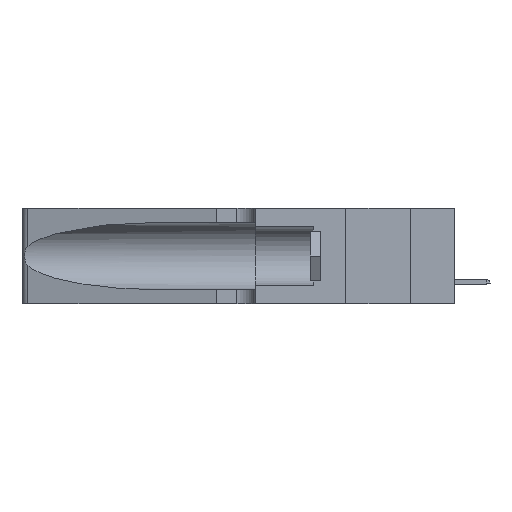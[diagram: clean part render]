
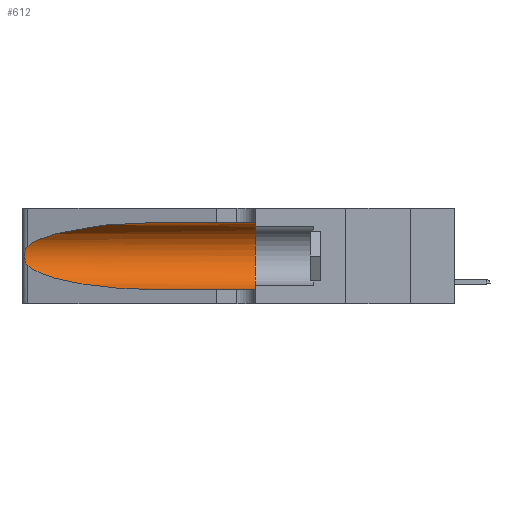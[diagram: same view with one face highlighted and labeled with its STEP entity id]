
A CAD part, left-side view. The second image highlights one B-rep face of the part: STEP entity #612.
In plain terms, the highlighted cylindrical face has radius 3.308 mm (diameter 6.617 mm), a partial arc.
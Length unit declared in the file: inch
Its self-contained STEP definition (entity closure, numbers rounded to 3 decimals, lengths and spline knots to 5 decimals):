
#334 = CARTESIAN_POINT ( 'NONE',  ( 0.26018, 1.23835, 0.19895 ) ) ;
#444 = CYLINDRICAL_SURFACE ( 'NONE', #19863, 0.13025 ) ;
#612 = ADVANCED_FACE ( 'NONE', ( #15831 ), #444, .F. ) ;
#922 = CARTESIAN_POINT ( 'NONE',  ( 0.25555, 1.22993, 0.14849 ) ) ;
#1124 = CARTESIAN_POINT ( 'NONE',  ( 0.25639, 1.23186, 0.15144 ) ) ;
#1495 = CARTESIAN_POINT ( 'NONE',  ( 0.18966, 0.96281, 0.05475 ) ) ;
#1857 = CARTESIAN_POINT ( 'NONE',  ( 0.25854, 1.2359, 0.20912 ) ) ;
#2413 = DIRECTION ( 'NONE',  ( 0., -1., 0. ) ) ;
#3185 = EDGE_CURVE ( 'NONE', #13664, #7599, #10979, .T. ) ;
#4632 = DIRECTION ( 'NONE',  ( 0., 0., -1. ) ) ;
#4920 = EDGE_CURVE ( 'NONE', #14132, #12364, #19684, .T. ) ;
#5044 = CARTESIAN_POINT ( 'NONE',  ( 0.26075, 1.23896, 0.178 ) ) ;
#5285 = CARTESIAN_POINT ( 'NONE',  ( 0.18966, 0.96281, 0.31525 ) ) ;
#5530 = ORIENTED_EDGE ( 'NONE', *, *, #4920, .T. ) ;
#5553 = VECTOR ( 'NONE', #2413, 39.37008 ) ;
#5659 =( BOUNDED_CURVE ( )  B_SPLINE_CURVE ( 3, ( #7695, #5937, #1495, #12233 ),
 .UNSPECIFIED., .F., .F. ) 
 B_SPLINE_CURVE_WITH_KNOTS ( ( 4, 4 ),
 ( 3.44316, 4.71239 ),
 .UNSPECIFIED. ) 
 CURVE ( )  GEOMETRIC_REPRESENTATION_ITEM ( )  RATIONAL_B_SPLINE_CURVE ( ( 1., 0.87, 0.87, 1. ) ) 
 REPRESENTATION_ITEM ( '' )  );
#5937 = CARTESIAN_POINT ( 'NONE',  ( 0.2373, 1.15595, 0.08982 ) ) ;
#6604 = CARTESIAN_POINT ( 'NONE',  ( 0.26075, 1.23896, 0.19203 ) ) ;
#6623 = ORIENTED_EDGE ( 'NONE', *, *, #3185, .F. ) ;
#6939 = CARTESIAN_POINT ( 'NONE',  ( 0.2373, 1.15595, 0.28018 ) ) ;
#7080 = VERTEX_POINT ( 'NONE', #13266 ) ;
#7240 = ORIENTED_EDGE ( 'NONE', *, *, #14362, .T. ) ;
#7599 = VERTEX_POINT ( 'NONE', #12850 ) ;
#7695 = CARTESIAN_POINT ( 'NONE',  ( 0.25487, 1.22718, 0.14631 ) ) ;
#7906 = ORIENTED_EDGE ( 'NONE', *, *, #10298, .T. ) ;
#8017 = AXIS2_PLACEMENT_3D ( 'NONE', #13587, #19824, #10641 ) ;
#8068 = CARTESIAN_POINT ( 'NONE',  ( 0.1305, 1.61858, 0.185 ) ) ;
#9756 = VERTEX_POINT ( 'NONE', #18602 ) ;
#9932 = CARTESIAN_POINT ( 'NONE',  ( 0.25555, 1.22994, 0.2215 ) ) ;
#10061 = CARTESIAN_POINT ( 'NONE',  ( 0.25487, 1.22718, 0.22369 ) ) ;
#10298 = EDGE_CURVE ( 'NONE', #12364, #9756, #18409, .T. ) ;
#10338 = ORIENTED_EDGE ( 'NONE', *, *, #15326, .T. ) ;
#10390 = CARTESIAN_POINT ( 'NONE',  ( 0.1305, 1.61858, 0.05475 ) ) ;
#10522 = LINE ( 'NONE', #19706, #20082 ) ;
#10641 = DIRECTION ( 'NONE',  ( 0., 0., 1. ) ) ;
#10655 = CARTESIAN_POINT ( 'NONE',  ( 0.25487, 1.22718, 0.14631 ) ) ;
#10979 = CIRCLE ( 'NONE', #8017, 0.13025 ) ;
#11494 = CARTESIAN_POINT ( 'NONE',  ( 0.1305, 0.72297, 0.31525 ) ) ;
#11836 = DIRECTION ( 'NONE',  ( 0., -1., 0. ) ) ;
#11866 = CARTESIAN_POINT ( 'NONE',  ( 0.25856, 1.23593, 0.16098 ) ) ;
#12233 = CARTESIAN_POINT ( 'NONE',  ( 0.1305, 0.72297, 0.05475 ) ) ;
#12364 = VERTEX_POINT ( 'NONE', #16515 ) ;
#12544 = CARTESIAN_POINT ( 'NONE',  ( 0.1305, 0.35, 0.31525 ) ) ;
#12850 = CARTESIAN_POINT ( 'NONE',  ( 0.1305, 0.35, 0.05475 ) ) ;
#13184 = CARTESIAN_POINT ( 'NONE',  ( 0.25787, 1.23484, 0.2124 ) ) ;
#13266 = CARTESIAN_POINT ( 'NONE',  ( 0.1305, 0.72297, 0.05475 ) ) ;
#13587 = CARTESIAN_POINT ( 'NONE',  ( 0.1305, 0.35, 0.185 ) ) ;
#13664 = VERTEX_POINT ( 'NONE', #12544 ) ;
#13961 = EDGE_CURVE ( 'NONE', #14132, #13664, #10522, .T. ) ;
#14132 = VERTEX_POINT ( 'NONE', #17641 ) ;
#14362 = EDGE_CURVE ( 'NONE', #7080, #7599, #19481, .T. ) ;
#15066 = CARTESIAN_POINT ( 'NONE',  ( 0.25789, 1.23486, 0.15765 ) ) ;
#15326 = EDGE_CURVE ( 'NONE', #9756, #7080, #5659, .T. ) ;
#15831 = FACE_OUTER_BOUND ( 'NONE', #17418, .T. ) ;
#16039 = CARTESIAN_POINT ( 'NONE',  ( 0.25487, 1.22718, 0.22369 ) ) ;
#16515 = CARTESIAN_POINT ( 'NONE',  ( 0.25487, 1.22718, 0.22369 ) ) ;
#16988 = ORIENTED_EDGE ( 'NONE', *, *, #13961, .F. ) ;
#17418 = EDGE_LOOP ( 'NONE', ( #5530, #7906, #10338, #7240, #6623, #16988 ) ) ;
#17641 = CARTESIAN_POINT ( 'NONE',  ( 0.1305, 0.72297, 0.31525 ) ) ;
#17705 = CARTESIAN_POINT ( 'NONE',  ( 0.26017, 1.23833, 0.17102 ) ) ;
#18409 = B_SPLINE_CURVE_WITH_KNOTS ( 'NONE', 3,
 ( #16039, #9932, #19432, #13184, #1857, #334, #6604, #5044, #17705, #11866, #15066, #1124, #922, #10655 ),
 .UNSPECIFIED., .F., .F.,
 ( 4, 2, 2, 2, 2, 2, 4 ),
 ( 0., 0.00027, 0.00053, 0.00107, 0.0016, 0.00187, 0.00214 ),
 .UNSPECIFIED. ) ;
#18602 = CARTESIAN_POINT ( 'NONE',  ( 0.25487, 1.22718, 0.14631 ) ) ;
#18833 = DIRECTION ( 'NONE',  ( 0., -1., 0. ) ) ;
#19432 = CARTESIAN_POINT ( 'NONE',  ( 0.25639, 1.23184, 0.21858 ) ) ;
#19481 = LINE ( 'NONE', #10390, #5553 ) ;
#19684 =( BOUNDED_CURVE ( )  B_SPLINE_CURVE ( 3, ( #11494, #5285, #6939, #10061 ),
 .UNSPECIFIED., .F., .F. ) 
 B_SPLINE_CURVE_WITH_KNOTS ( ( 4, 4 ),
 ( 1.5708, 2.84003 ),
 .UNSPECIFIED. ) 
 CURVE ( )  GEOMETRIC_REPRESENTATION_ITEM ( )  RATIONAL_B_SPLINE_CURVE ( ( 1., 0.87, 0.87, 1. ) ) 
 REPRESENTATION_ITEM ( '' )  );
#19706 = CARTESIAN_POINT ( 'NONE',  ( 0.1305, 1.61858, 0.31525 ) ) ;
#19824 = DIRECTION ( 'NONE',  ( 0., 1., 0. ) ) ;
#19863 = AXIS2_PLACEMENT_3D ( 'NONE', #8068, #18833, #4632 ) ;
#20082 = VECTOR ( 'NONE', #11836, 39.37008 ) ;
